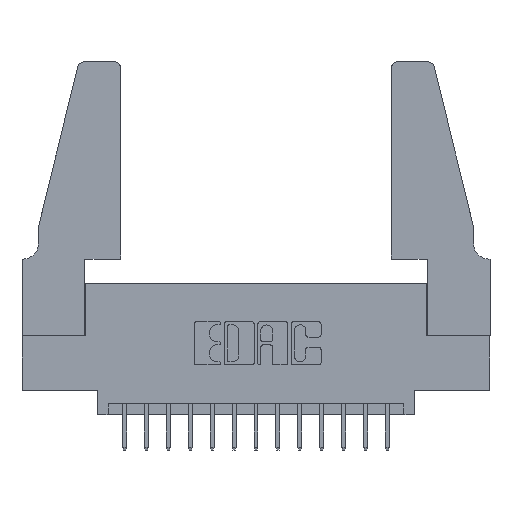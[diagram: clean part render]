
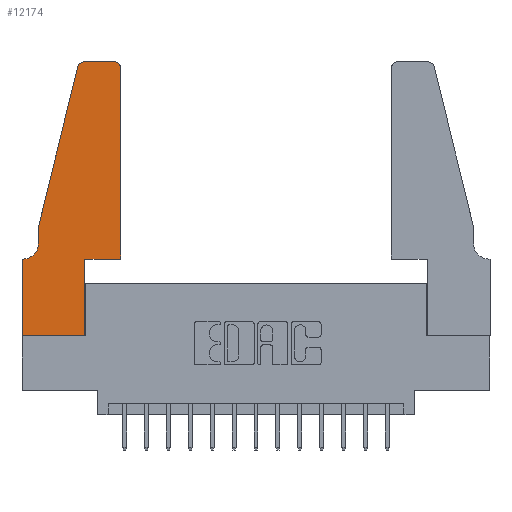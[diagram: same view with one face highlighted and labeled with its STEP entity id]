
A CAD part, top view. The second image highlights one B-rep face of the part: STEP entity #12174.
In plain terms, the highlighted planar face has unit normal (0, 0, 1).
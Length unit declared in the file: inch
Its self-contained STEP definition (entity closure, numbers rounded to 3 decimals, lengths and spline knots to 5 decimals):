
#344 = EDGE_CURVE ( 'NONE', #9720, #1586, #12570, .T. ) ;
#455 = VERTEX_POINT ( 'NONE', #9124 ) ;
#588 = EDGE_CURVE ( 'NONE', #8436, #455, #6557, .T. ) ;
#803 = LINE ( 'NONE', #5152, #10678 ) ;
#1067 = AXIS2_PLACEMENT_3D ( 'NONE', #1107, #1159, #1131 ) ;
#1107 = CARTESIAN_POINT ( 'NONE',  ( 0.284, 1.22, 0.37 ) ) ;
#1131 = DIRECTION ( 'NONE',  ( 1., 0., 0. ) ) ;
#1159 = DIRECTION ( 'NONE',  ( 0., 0., 1. ) ) ;
#1267 = ORIENTED_EDGE ( 'NONE', *, *, #16071, .T. ) ;
#1276 = CARTESIAN_POINT ( 'NONE',  ( 0., 0., 0.37 ) ) ;
#1427 = ORIENTED_EDGE ( 'NONE', *, *, #13439, .T. ) ;
#1586 = VERTEX_POINT ( 'NONE', #4507 ) ;
#1824 = ORIENTED_EDGE ( 'NONE', *, *, #9747, .T. ) ;
#1830 = LINE ( 'NONE', #13792, #15231 ) ;
#1879 = VERTEX_POINT ( 'NONE', #4156 ) ;
#1923 = ORIENTED_EDGE ( 'NONE', *, *, #13786, .T. ) ;
#2030 = CARTESIAN_POINT ( 'NONE',  ( 0., 0., 0.37 ) ) ;
#2070 = CARTESIAN_POINT ( 'NONE',  ( 0.0755, 0.5, 0.37 ) ) ;
#2242 = VECTOR ( 'NONE', #11619, 39.37008 ) ;
#2440 = CARTESIAN_POINT ( 'NONE',  ( 0.0755, 0.5, 0.37 ) ) ;
#2523 = VECTOR ( 'NONE', #10068, 39.37008 ) ;
#2535 = CARTESIAN_POINT ( 'NONE',  ( 0.0755, 0.42, 0.37 ) ) ;
#2927 = EDGE_CURVE ( 'NONE', #14015, #5206, #9080, .T. ) ;
#2992 = VECTOR ( 'NONE', #13937, 39.37008 ) ;
#3106 = VERTEX_POINT ( 'NONE', #6834 ) ;
#3268 = ORIENTED_EDGE ( 'NONE', *, *, #6172, .T. ) ;
#3498 = CARTESIAN_POINT ( 'NONE',  ( 0.2865, 0.35, 0.37 ) ) ;
#3684 = CARTESIAN_POINT ( 'NONE',  ( 0.4505, 0.35, 0.37 ) ) ;
#3725 = CARTESIAN_POINT ( 'NONE',  ( 0.2605, 1.25, 0.37 ) ) ;
#3887 = VECTOR ( 'NONE', #12511, 39.37008 ) ;
#4156 = CARTESIAN_POINT ( 'NONE',  ( 0., 0.35, 0.37 ) ) ;
#4215 = CIRCLE ( 'NONE', #12859, 0.03 ) ;
#4280 = ORIENTED_EDGE ( 'NONE', *, *, #5871, .T. ) ;
#4507 = CARTESIAN_POINT ( 'NONE',  ( 0.4505, 1.22, 0.37 ) ) ;
#4724 = CARTESIAN_POINT ( 'NONE',  ( 0.4205, 1.22, 0.37 ) ) ;
#4865 = VERTEX_POINT ( 'NONE', #2070 ) ;
#5152 = CARTESIAN_POINT ( 'NONE',  ( 0.4505, 0.35, 0.37 ) ) ;
#5206 = VERTEX_POINT ( 'NONE', #7894 ) ;
#5221 = ORIENTED_EDGE ( 'NONE', *, *, #344, .T. ) ;
#5301 = CARTESIAN_POINT ( 'NONE',  ( 0.0755, 0.35, 0.37 ) ) ;
#5306 = LINE ( 'NONE', #3498, #14071 ) ;
#5687 = LINE ( 'NONE', #5301, #2242 ) ;
#5827 = ORIENTED_EDGE ( 'NONE', *, *, #588, .T. ) ;
#5871 = EDGE_CURVE ( 'NONE', #5206, #1879, #5687, .T. ) ;
#5985 = DIRECTION ( 'NONE',  ( 1., 0., 0. ) ) ;
#6167 = CARTESIAN_POINT ( 'NONE',  ( 0.2865, 0.35, 0.37 ) ) ;
#6169 = CARTESIAN_POINT ( 'NONE',  ( 0., 0.35, 0.37 ) ) ;
#6172 = EDGE_CURVE ( 'NONE', #1879, #12450, #10959, .T. ) ;
#6557 = CIRCLE ( 'NONE', #1067, 0.03 ) ;
#6834 = CARTESIAN_POINT ( 'NONE',  ( 0.4205, 1.25, 0.37 ) ) ;
#7585 = DIRECTION ( 'NONE',  ( -1., 0., 0. ) ) ;
#7695 = VECTOR ( 'NONE', #12193, 39.37008 ) ;
#7894 = CARTESIAN_POINT ( 'NONE',  ( 0.0055, 0.35, 0.37 ) ) ;
#8059 = EDGE_CURVE ( 'NONE', #3106, #8436, #16287, .T. ) ;
#8069 = ORIENTED_EDGE ( 'NONE', *, *, #8059, .T. ) ;
#8277 = CARTESIAN_POINT ( 'NONE',  ( 0.2865, 0., 0.37 ) ) ;
#8436 = VERTEX_POINT ( 'NONE', #9496 ) ;
#8556 = ORIENTED_EDGE ( 'NONE', *, *, #10240, .T. ) ;
#8627 = DIRECTION ( 'NONE',  ( -1., 0., 0. ) ) ;
#8644 = DIRECTION ( 'NONE',  ( 0., 0., -1. ) ) ;
#8681 = CARTESIAN_POINT ( 'NONE',  ( 0.0055, 0.42, 0.37 ) ) ;
#8729 = DIRECTION ( 'NONE',  ( 1., 0., 0. ) ) ;
#9080 = CIRCLE ( 'NONE', #16141, 0.07 ) ;
#9124 = CARTESIAN_POINT ( 'NONE',  ( 0.25487, 1.22718, 0.37 ) ) ;
#9496 = CARTESIAN_POINT ( 'NONE',  ( 0.284, 1.25, 0.37 ) ) ;
#9720 = VERTEX_POINT ( 'NONE', #3684 ) ;
#9746 = VECTOR ( 'NONE', #7585, 39.37008 ) ;
#9747 = EDGE_CURVE ( 'NONE', #4865, #14015, #1830, .T. ) ;
#10018 = CARTESIAN_POINT ( 'NONE',  ( 0.4505, 0.35, 0.37 ) ) ;
#10068 = DIRECTION ( 'NONE',  ( 0., 1., 0. ) ) ;
#10132 = LINE ( 'NONE', #1276, #2992 ) ;
#10240 = EDGE_CURVE ( 'NONE', #14309, #10307, #5306, .T. ) ;
#10307 = VERTEX_POINT ( 'NONE', #6167 ) ;
#10678 = VECTOR ( 'NONE', #15049, 39.37008 ) ;
#10946 = LINE ( 'NONE', #2440, #3887 ) ;
#10959 = LINE ( 'NONE', #2030, #7695 ) ;
#11619 = DIRECTION ( 'NONE',  ( -1., 0., 0. ) ) ;
#11888 = FACE_OUTER_BOUND ( 'NONE', #13245, .T. ) ;
#12174 = ADVANCED_FACE ( 'NONE', ( #11888 ), #14859, .T. ) ;
#12193 = DIRECTION ( 'NONE',  ( 0., -1., 0. ) ) ;
#12234 = DIRECTION ( 'NONE',  ( 0., 1., 0. ) ) ;
#12450 = VERTEX_POINT ( 'NONE', #15835 ) ;
#12511 = DIRECTION ( 'NONE',  ( -0.239, -0.971, 0. ) ) ;
#12570 = LINE ( 'NONE', #10018, #2523 ) ;
#12696 = ORIENTED_EDGE ( 'NONE', *, *, #2927, .T. ) ;
#12733 = AXIS2_PLACEMENT_3D ( 'NONE', #6169, #16085, #8729 ) ;
#12859 = AXIS2_PLACEMENT_3D ( 'NONE', #4724, #13445, #5985 ) ;
#13245 = EDGE_LOOP ( 'NONE', ( #8069, #5827, #1267, #1824, #12696, #4280, #3268, #1427, #8556, #13977, #5221, #1923 ) ) ;
#13439 = EDGE_CURVE ( 'NONE', #12450, #14309, #10132, .T. ) ;
#13445 = DIRECTION ( 'NONE',  ( 0., 0., 1. ) ) ;
#13786 = EDGE_CURVE ( 'NONE', #1586, #3106, #4215, .T. ) ;
#13792 = CARTESIAN_POINT ( 'NONE',  ( 0.0755, 0.5, 0.37 ) ) ;
#13937 = DIRECTION ( 'NONE',  ( 1., 0., 0. ) ) ;
#13977 = ORIENTED_EDGE ( 'NONE', *, *, #14022, .T. ) ;
#14015 = VERTEX_POINT ( 'NONE', #2535 ) ;
#14022 = EDGE_CURVE ( 'NONE', #10307, #9720, #803, .T. ) ;
#14071 = VECTOR ( 'NONE', #12234, 39.37008 ) ;
#14309 = VERTEX_POINT ( 'NONE', #8277 ) ;
#14859 = PLANE ( 'NONE',  #12733 ) ;
#15023 = DIRECTION ( 'NONE',  ( 0., -1., 0. ) ) ;
#15049 = DIRECTION ( 'NONE',  ( 1., 0., 0. ) ) ;
#15231 = VECTOR ( 'NONE', #15023, 39.37008 ) ;
#15835 = CARTESIAN_POINT ( 'NONE',  ( 0., 0., 0.37 ) ) ;
#16071 = EDGE_CURVE ( 'NONE', #455, #4865, #10946, .T. ) ;
#16085 = DIRECTION ( 'NONE',  ( 0., 0., 1. ) ) ;
#16141 = AXIS2_PLACEMENT_3D ( 'NONE', #8681, #8644, #8627 ) ;
#16287 = LINE ( 'NONE', #3725, #9746 ) ;
